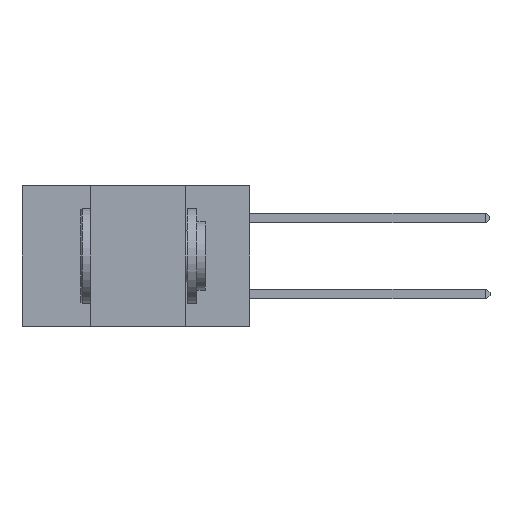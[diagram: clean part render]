
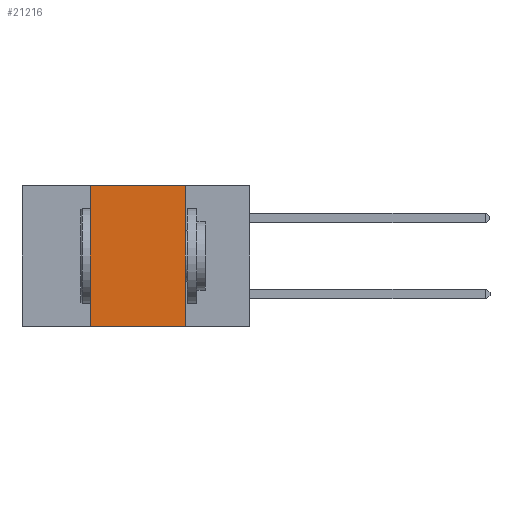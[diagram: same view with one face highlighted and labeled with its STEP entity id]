
A CAD part, left-side view. The second image highlights one B-rep face of the part: STEP entity #21216.
In plain terms, the highlighted planar face has unit normal (-1, 0, 0).
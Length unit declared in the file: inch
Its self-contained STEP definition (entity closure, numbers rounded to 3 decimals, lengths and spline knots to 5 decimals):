
#532 = DIRECTION ( 'NONE',  ( 0., -1., 0. ) ) ;
#842 = DIRECTION ( 'NONE',  ( 0., -1., 0. ) ) ;
#1196 = CARTESIAN_POINT ( 'NONE',  ( 0., 0.42, 0. ) ) ;
#1259 = DIRECTION ( 'NONE',  ( 0., 0., -1. ) ) ;
#1478 = ORIENTED_EDGE ( 'NONE', *, *, #17500, .F. ) ;
#5732 = VECTOR ( 'NONE', #532, 39.37008 ) ;
#6495 = CARTESIAN_POINT ( 'NONE',  ( 0., 0.42, 0. ) ) ;
#6790 = LINE ( 'NONE', #11263, #20810 ) ;
#6798 = EDGE_LOOP ( 'NONE', ( #21205, #1478, #12817, #21770 ) ) ;
#7078 = CARTESIAN_POINT ( 'NONE',  ( 0., 0.42, -0.37 ) ) ;
#8080 = PLANE ( 'NONE',  #8543 ) ;
#8098 = LINE ( 'NONE', #17324, #17011 ) ;
#8474 = DIRECTION ( 'NONE',  ( 0., 0., -1. ) ) ;
#8543 = AXIS2_PLACEMENT_3D ( 'NONE', #22172, #11698, #1259 ) ;
#10403 = LINE ( 'NONE', #12389, #5732 ) ;
#10562 = EDGE_CURVE ( 'NONE', #13636, #21924, #19502, .T. ) ;
#10631 = FACE_OUTER_BOUND ( 'NONE', #6798, .T. ) ;
#10745 = EDGE_CURVE ( 'NONE', #13636, #18096, #10403, .T. ) ;
#11263 = CARTESIAN_POINT ( 'NONE',  ( 0., 0.6, 0. ) ) ;
#11698 = DIRECTION ( 'NONE',  ( 1., 0., 0. ) ) ;
#11770 = EDGE_CURVE ( 'NONE', #15074, #18096, #8098, .T. ) ;
#12389 = CARTESIAN_POINT ( 'NONE',  ( 0., 0.6, -0.37 ) ) ;
#12817 = ORIENTED_EDGE ( 'NONE', *, *, #10562, .F. ) ;
#13636 = VERTEX_POINT ( 'NONE', #7078 ) ;
#15074 = VERTEX_POINT ( 'NONE', #18387 ) ;
#17011 = VECTOR ( 'NONE', #8474, 39.37008 ) ;
#17324 = CARTESIAN_POINT ( 'NONE',  ( 0., 0.17, 0. ) ) ;
#17500 = EDGE_CURVE ( 'NONE', #21924, #15074, #6790, .T. ) ;
#18096 = VERTEX_POINT ( 'NONE', #19760 ) ;
#18387 = CARTESIAN_POINT ( 'NONE',  ( 0., 0.17, 0. ) ) ;
#18701 = DIRECTION ( 'NONE',  ( 0., 0., 1. ) ) ;
#18960 = VECTOR ( 'NONE', #18701, 39.37008 ) ;
#19502 = LINE ( 'NONE', #1196, #18960 ) ;
#19760 = CARTESIAN_POINT ( 'NONE',  ( 0., 0.17, -0.37 ) ) ;
#20810 = VECTOR ( 'NONE', #842, 39.37008 ) ;
#21205 = ORIENTED_EDGE ( 'NONE', *, *, #11770, .F. ) ;
#21216 = ADVANCED_FACE ( 'NONE', ( #10631 ), #8080, .F. ) ;
#21770 = ORIENTED_EDGE ( 'NONE', *, *, #10745, .T. ) ;
#21924 = VERTEX_POINT ( 'NONE', #6495 ) ;
#22172 = CARTESIAN_POINT ( 'NONE',  ( 0., 0.6, 0. ) ) ;
